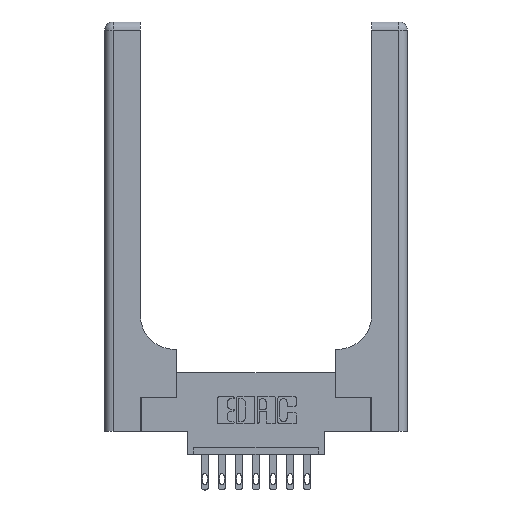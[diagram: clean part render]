
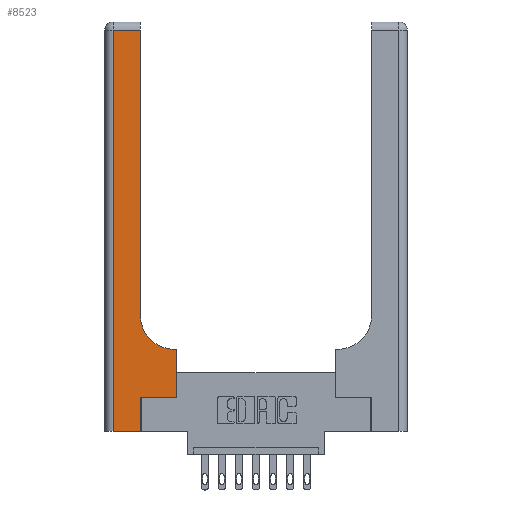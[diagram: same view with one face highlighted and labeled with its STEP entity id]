
A CAD part, top view. The second image highlights one B-rep face of the part: STEP entity #8523.
In plain terms, the highlighted planar face has unit normal (0, 0, 1).
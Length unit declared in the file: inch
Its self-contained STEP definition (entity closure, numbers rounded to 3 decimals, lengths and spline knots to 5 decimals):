
#58 = VECTOR ( 'NONE', #13283, 39.37008 ) ;
#297 = LINE ( 'NONE', #6252, #10998 ) ;
#468 = EDGE_CURVE ( 'NONE', #13924, #1447, #14182, .T. ) ;
#507 = DIRECTION ( 'NONE',  ( 1., 0., 0. ) ) ;
#863 = EDGE_LOOP ( 'NONE', ( #8573, #8409, #14686, #4005, #1165, #10129, #11094, #4413, #11812 ) ) ;
#1003 = LINE ( 'NONE', #12192, #10959 ) ;
#1165 = ORIENTED_EDGE ( 'NONE', *, *, #3320, .T. ) ;
#1447 = VERTEX_POINT ( 'NONE', #5540 ) ;
#1457 = DIRECTION ( 'NONE',  ( -1., 0., 0. ) ) ;
#1539 = DIRECTION ( 'NONE',  ( 0., 0., -1. ) ) ;
#1931 = DIRECTION ( 'NONE',  ( 0., 1., 0. ) ) ;
#2274 = CARTESIAN_POINT ( 'NONE',  ( 0.26, 0.6, 0.37 ) ) ;
#2363 = CARTESIAN_POINT ( 'NONE',  ( 0.528, 0.25, 0.37 ) ) ;
#2585 = VECTOR ( 'NONE', #1931, 39.37008 ) ;
#3083 = DIRECTION ( 'NONE',  ( 0., 1., 0. ) ) ;
#3175 = DIRECTION ( 'NONE',  ( -1., 0., 0. ) ) ;
#3320 = EDGE_CURVE ( 'NONE', #7534, #14691, #5083, .T. ) ;
#3395 = LINE ( 'NONE', #2274, #4789 ) ;
#3812 = VECTOR ( 'NONE', #12342, 39.37008 ) ;
#4005 = ORIENTED_EDGE ( 'NONE', *, *, #13837, .T. ) ;
#4413 = ORIENTED_EDGE ( 'NONE', *, *, #13907, .T. ) ;
#4760 = FACE_OUTER_BOUND ( 'NONE', #863, .T. ) ;
#4789 = VECTOR ( 'NONE', #3175, 39.37008 ) ;
#4903 = PLANE ( 'NONE',  #7717 ) ;
#5083 = LINE ( 'NONE', #9641, #58 ) ;
#5136 = AXIS2_PLACEMENT_3D ( 'NONE', #10813, #1539, #12897 ) ;
#5258 = VECTOR ( 'NONE', #9613, 39.37008 ) ;
#5325 = VERTEX_POINT ( 'NONE', #6790 ) ;
#5371 = EDGE_CURVE ( 'NONE', #14691, #12567, #297, .T. ) ;
#5451 = EDGE_CURVE ( 'NONE', #5325, #14272, #12752, .T. ) ;
#5491 = LINE ( 'NONE', #6834, #3812 ) ;
#5540 = CARTESIAN_POINT ( 'NONE',  ( 0.26, 0.85, 0.37 ) ) ;
#5988 = CARTESIAN_POINT ( 'NONE',  ( 0.528, 0.6, 0.37 ) ) ;
#6019 = LINE ( 'NONE', #13849, #6137 ) ;
#6137 = VECTOR ( 'NONE', #1457, 39.37008 ) ;
#6147 = CARTESIAN_POINT ( 'NONE',  ( 0.265, 0.25, 0.37 ) ) ;
#6252 = CARTESIAN_POINT ( 'NONE',  ( 0.265, 0.25, 0.37 ) ) ;
#6381 = CARTESIAN_POINT ( 'NONE',  ( 0.26, 2.94, 0.37 ) ) ;
#6611 = CARTESIAN_POINT ( 'NONE',  ( 0.51, 0.6, 0.37 ) ) ;
#6790 = CARTESIAN_POINT ( 'NONE',  ( 0.06, 2.94, 0.37 ) ) ;
#6834 = CARTESIAN_POINT ( 'NONE',  ( 0., 0., 0.37 ) ) ;
#7134 = CARTESIAN_POINT ( 'NONE',  ( 0., 3., 0.37 ) ) ;
#7534 = VERTEX_POINT ( 'NONE', #9880 ) ;
#7717 = AXIS2_PLACEMENT_3D ( 'NONE', #7134, #13844, #8105 ) ;
#7756 = CARTESIAN_POINT ( 'NONE',  ( 0.26, 3., 0.37 ) ) ;
#8105 = DIRECTION ( 'NONE',  ( -1., 0., 0. ) ) ;
#8409 = ORIENTED_EDGE ( 'NONE', *, *, #11295, .T. ) ;
#8523 = ADVANCED_FACE ( 'NONE', ( #4760 ), #4903, .F. ) ;
#8573 = ORIENTED_EDGE ( 'NONE', *, *, #9560, .T. ) ;
#8784 = EDGE_CURVE ( 'NONE', #12567, #13960, #1003, .T. ) ;
#9560 = EDGE_CURVE ( 'NONE', #1447, #11406, #10069, .T. ) ;
#9613 = DIRECTION ( 'NONE',  ( 0., -1., 0. ) ) ;
#9641 = CARTESIAN_POINT ( 'NONE',  ( 0.265, 0., 0.37 ) ) ;
#9880 = CARTESIAN_POINT ( 'NONE',  ( 0.265, 0., 0.37 ) ) ;
#10069 = LINE ( 'NONE', #7756, #2585 ) ;
#10129 = ORIENTED_EDGE ( 'NONE', *, *, #5371, .T. ) ;
#10735 = CARTESIAN_POINT ( 'NONE',  ( 0.06, 3., 0.37 ) ) ;
#10813 = CARTESIAN_POINT ( 'NONE',  ( 0.51, 0.85, 0.37 ) ) ;
#10959 = VECTOR ( 'NONE', #3083, 39.37008 ) ;
#10998 = VECTOR ( 'NONE', #507, 39.37008 ) ;
#11094 = ORIENTED_EDGE ( 'NONE', *, *, #8784, .T. ) ;
#11295 = EDGE_CURVE ( 'NONE', #11406, #5325, #6019, .T. ) ;
#11406 = VERTEX_POINT ( 'NONE', #6381 ) ;
#11812 = ORIENTED_EDGE ( 'NONE', *, *, #468, .T. ) ;
#12192 = CARTESIAN_POINT ( 'NONE',  ( 0.528, 0.25, 0.37 ) ) ;
#12342 = DIRECTION ( 'NONE',  ( 1., 0., 0. ) ) ;
#12567 = VERTEX_POINT ( 'NONE', #2363 ) ;
#12752 = LINE ( 'NONE', #10735, #5258 ) ;
#12897 = DIRECTION ( 'NONE',  ( 1., 0., 0. ) ) ;
#13283 = DIRECTION ( 'NONE',  ( 0., 1., 0. ) ) ;
#13837 = EDGE_CURVE ( 'NONE', #14272, #7534, #5491, .T. ) ;
#13844 = DIRECTION ( 'NONE',  ( 0., 0., -1. ) ) ;
#13849 = CARTESIAN_POINT ( 'NONE',  ( 0., 2.94, 0.37 ) ) ;
#13862 = CARTESIAN_POINT ( 'NONE',  ( 0.06, 0., 0.37 ) ) ;
#13907 = EDGE_CURVE ( 'NONE', #13960, #13924, #3395, .T. ) ;
#13924 = VERTEX_POINT ( 'NONE', #6611 ) ;
#13960 = VERTEX_POINT ( 'NONE', #5988 ) ;
#14182 = CIRCLE ( 'NONE', #5136, 0.25 ) ;
#14272 = VERTEX_POINT ( 'NONE', #13862 ) ;
#14686 = ORIENTED_EDGE ( 'NONE', *, *, #5451, .T. ) ;
#14691 = VERTEX_POINT ( 'NONE', #6147 ) ;
